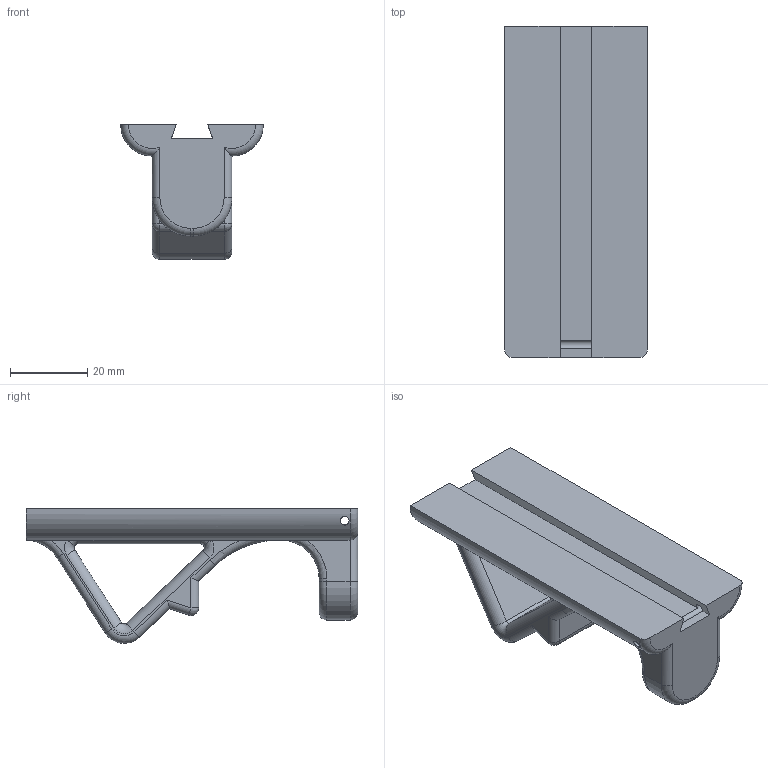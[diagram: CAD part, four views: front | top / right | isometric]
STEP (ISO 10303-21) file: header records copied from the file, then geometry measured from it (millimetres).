
FILE_DESCRIPTION(/* description */ (''),/* implementation_level */ '2;1');
FILE_NAME(/* name */ 'Shorty Handstop v10 - AFG.step',/* time_stamp */ '2020-06-28T23:18:03-04:00',/* author */ (''),/* organization */ (''),/* preprocessor_version */ 'ST-DEVELOPER v18.1',/* originating_system */ 'Autodesk Translation Framework v9.3.0.1241',/* authorisation */ '');
FILE_SCHEMA (('AUTOMOTIVE_DESIGN { 1 0 10303 214 3 1 1 }'));
Length unit declared in the file: millimetre
Products named in the file (1): Shorty Handstop
Bounding box: 37 x 86 x 34.95 mm (x, y, z)
Volume: 32978.1 mm3; surface area: 12575.9 mm2
Topology: 1 solids, 1 shells, 84 faces, 210 edges, 124 vertices
Faces by surface type: cylinder 35, torus 24, plane 23, sphere 2
Full cylindrical faces by diameter (mm): 2.25 x1
Entity records: 2661 total; most frequent: CARTESIAN_POINT 585, DIRECTION 458, ORIENTED_EDGE 420, EDGE_CURVE 210, AXIS2_PLACEMENT_3D 181, VERTEX_POINT 124, LINE 96, VECTOR 96
